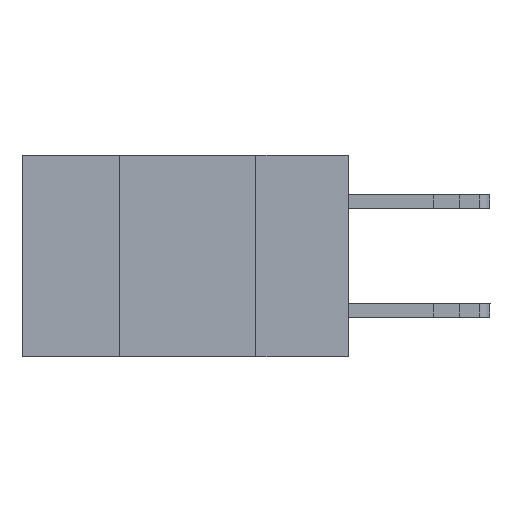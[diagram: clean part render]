
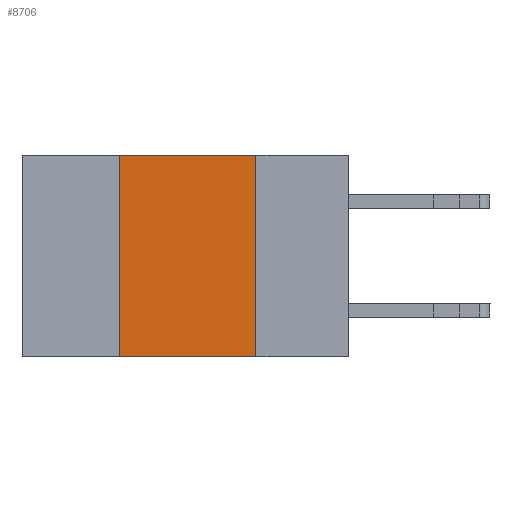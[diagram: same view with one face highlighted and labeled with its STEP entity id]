
A CAD part, left-side view. The second image highlights one B-rep face of the part: STEP entity #8706.
In plain terms, the highlighted planar face has unit normal (-1, 0, 0).
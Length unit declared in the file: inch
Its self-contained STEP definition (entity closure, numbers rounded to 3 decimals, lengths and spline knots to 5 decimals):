
#1012 = EDGE_CURVE ( 'NONE', #10040, #3233, #2463, .T. ) ;
#1400 = VERTEX_POINT ( 'NONE', #5474 ) ;
#1479 = DIRECTION ( 'NONE',  ( 0., 0., -1. ) ) ;
#1629 = EDGE_CURVE ( 'NONE', #9998, #1400, #9320, .T. ) ;
#1760 = CARTESIAN_POINT ( 'NONE',  ( 0., 0.42, 0. ) ) ;
#2463 = LINE ( 'NONE', #7897, #12085 ) ;
#3233 = VERTEX_POINT ( 'NONE', #3242 ) ;
#3242 = CARTESIAN_POINT ( 'NONE',  ( 0., 0.17, -0.37 ) ) ;
#3465 = DIRECTION ( 'NONE',  ( 0., -1., 0. ) ) ;
#3786 = FACE_OUTER_BOUND ( 'NONE', #6451, .T. ) ;
#3843 = LINE ( 'NONE', #10067, #12219 ) ;
#3893 = LINE ( 'NONE', #12747, #6690 ) ;
#4190 = VECTOR ( 'NONE', #12004, 39.37008 ) ;
#4684 = ORIENTED_EDGE ( 'NONE', *, *, #1012, .F. ) ;
#4799 = CARTESIAN_POINT ( 'NONE',  ( 0., 0.42, -0.37 ) ) ;
#5187 = EDGE_CURVE ( 'NONE', #1400, #10040, #3893, .T. ) ;
#5474 = CARTESIAN_POINT ( 'NONE',  ( 0., 0.42, 0. ) ) ;
#6451 = EDGE_LOOP ( 'NONE', ( #4684, #11419, #8305, #11025 ) ) ;
#6617 = PLANE ( 'NONE',  #8533 ) ;
#6690 = VECTOR ( 'NONE', #3465, 39.37008 ) ;
#6867 = CARTESIAN_POINT ( 'NONE',  ( 0., 0.17, 0. ) ) ;
#7739 = DIRECTION ( 'NONE',  ( 1., 0., 0. ) ) ;
#7897 = CARTESIAN_POINT ( 'NONE',  ( 0., 0.17, 0. ) ) ;
#8305 = ORIENTED_EDGE ( 'NONE', *, *, #1629, .F. ) ;
#8533 = AXIS2_PLACEMENT_3D ( 'NONE', #12724, #7739, #1479 ) ;
#8706 = ADVANCED_FACE ( 'NONE', ( #3786 ), #6617, .F. ) ;
#9082 = DIRECTION ( 'NONE',  ( 0., -1., 0. ) ) ;
#9320 = LINE ( 'NONE', #1760, #4190 ) ;
#9998 = VERTEX_POINT ( 'NONE', #4799 ) ;
#10040 = VERTEX_POINT ( 'NONE', #6867 ) ;
#10067 = CARTESIAN_POINT ( 'NONE',  ( 0., 0.6, -0.37 ) ) ;
#11002 = DIRECTION ( 'NONE',  ( 0., 0., -1. ) ) ;
#11025 = ORIENTED_EDGE ( 'NONE', *, *, #12793, .T. ) ;
#11419 = ORIENTED_EDGE ( 'NONE', *, *, #5187, .F. ) ;
#12004 = DIRECTION ( 'NONE',  ( 0., 0., 1. ) ) ;
#12085 = VECTOR ( 'NONE', #11002, 39.37008 ) ;
#12219 = VECTOR ( 'NONE', #9082, 39.37008 ) ;
#12724 = CARTESIAN_POINT ( 'NONE',  ( 0., 0.6, 0. ) ) ;
#12747 = CARTESIAN_POINT ( 'NONE',  ( 0., 0.6, 0. ) ) ;
#12793 = EDGE_CURVE ( 'NONE', #9998, #3233, #3843, .T. ) ;
